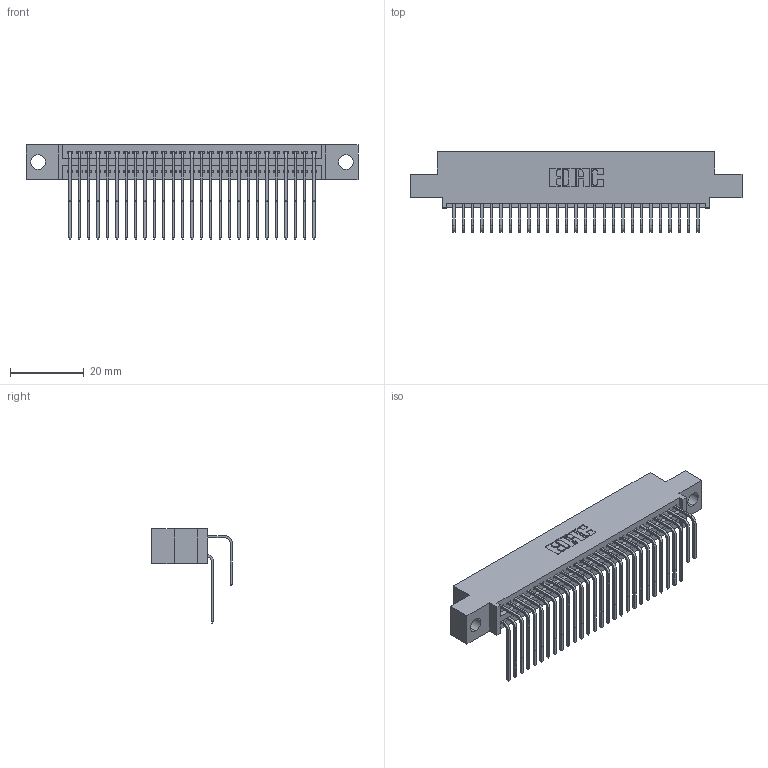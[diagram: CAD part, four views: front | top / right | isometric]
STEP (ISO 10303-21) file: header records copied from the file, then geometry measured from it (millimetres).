
FILE_DESCRIPTION (( 'STEP AP203' ), '1' );
FILE_NAME ('345-054-558-504.STEP', '2021-05-20T04:19:28', ( '' ), ( '' ), 'SwSTEP 2.0', 'SolidWorks 2020', '' );
FILE_SCHEMA (( 'CONFIG_CONTROL_DESIGN' ));
Length unit declared in the file: inch
Products named in the file (4): 345-054-558-504; 345-292-001_558 Tail - 2; 345 Part_0.110 Offset - 0.156 Dia-TI; 345-292-001_558 559 Tail - 1
Assembly tree (55 placements, depth 2):
  345-054-558-504
    345 Part_0.110 Offset - 0.156 Dia-TI
    345-292-001_558 559 Tail - 1  x27
    345-292-001_558 Tail - 2  x27
Bounding box: 89.79 x 21.83 x 25.53 mm (x, y, z)
Volume: 8715.2 mm3; surface area: 14001.2 mm2
Topology: 55 solids, 55 shells, 2952 faces, 8759 edges, 5766 vertices
Faces by surface type: plane 1988, cylinder 964
Entity records: 25407 total; most frequent: CARTESIAN_POINT 4325, ORIENTED_EDGE 4206, DIRECTION 3803, EDGE_CURVE 2103, LINE 1823, VECTOR 1823, VERTEX_POINT 1398, AXIS2_PLACEMENT_3D 990
